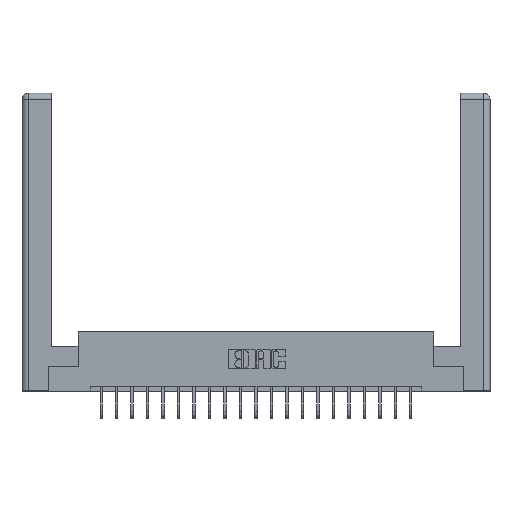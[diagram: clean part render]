
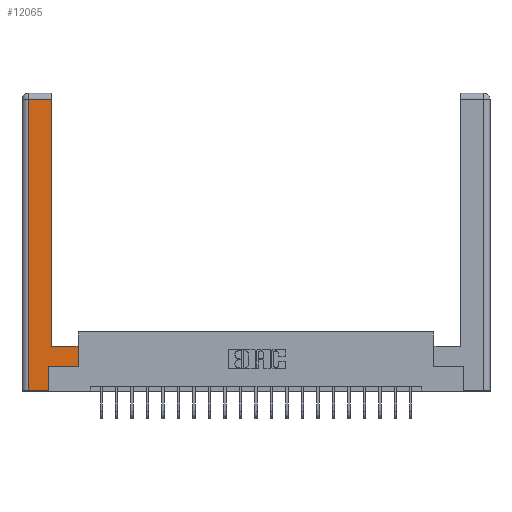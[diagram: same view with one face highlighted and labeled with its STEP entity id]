
A CAD part, top view. The second image highlights one B-rep face of the part: STEP entity #12065.
In plain terms, the highlighted planar face has unit normal (0, 0, 1).
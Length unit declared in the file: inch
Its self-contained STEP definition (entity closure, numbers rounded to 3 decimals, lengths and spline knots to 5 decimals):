
#113 = DIRECTION ( 'NONE',  ( 1., 0., 0. ) ) ;
#140 = CARTESIAN_POINT ( 'NONE',  ( 0.565, 0.45, 0. ) ) ;
#255 = PLANE ( 'NONE',  #15742 ) ;
#606 = CARTESIAN_POINT ( 'NONE',  ( 0.565, 0.245, 0. ) ) ;
#1697 = VERTEX_POINT ( 'NONE', #17633 ) ;
#1899 = VECTOR ( 'NONE', #22038, 39.37008 ) ;
#2042 = CARTESIAN_POINT ( 'NONE',  ( 0.265, 0.245, 0. ) ) ;
#2050 = CARTESIAN_POINT ( 'NONE',  ( 0.565, 0.245, 0. ) ) ;
#2191 = ORIENTED_EDGE ( 'NONE', *, *, #4860, .T. ) ;
#2798 = VECTOR ( 'NONE', #8363, 39.37008 ) ;
#2840 = LINE ( 'NONE', #2050, #11874 ) ;
#4106 = DIRECTION ( 'NONE',  ( 0., 0., -1. ) ) ;
#4717 = CARTESIAN_POINT ( 'NONE',  ( 0.0615, 0., 0. ) ) ;
#4752 = DIRECTION ( 'NONE',  ( 1., 0., 0. ) ) ;
#4832 = CARTESIAN_POINT ( 'NONE',  ( 0.265, 0.245, 0. ) ) ;
#4838 = VERTEX_POINT ( 'NONE', #606 ) ;
#4860 = EDGE_CURVE ( 'NONE', #20187, #1697, #8771, .T. ) ;
#6125 = DIRECTION ( 'NONE',  ( 0., 1., 0. ) ) ;
#6168 = EDGE_CURVE ( 'NONE', #13721, #4838, #2840, .T. ) ;
#6386 = VECTOR ( 'NONE', #6125, 39.37008 ) ;
#6642 = LINE ( 'NONE', #4717, #18558 ) ;
#7046 = ORIENTED_EDGE ( 'NONE', *, *, #20516, .T. ) ;
#7516 = LINE ( 'NONE', #4832, #6386 ) ;
#7944 = DIRECTION ( 'NONE',  ( 0., 1., 0. ) ) ;
#8049 = ORIENTED_EDGE ( 'NONE', *, *, #19619, .T. ) ;
#8363 = DIRECTION ( 'NONE',  ( -1., 0., 0. ) ) ;
#8366 = VERTEX_POINT ( 'NONE', #10975 ) ;
#8700 = EDGE_LOOP ( 'NONE', ( #2191, #8049, #17973, #20646, #8934, #20137, #7046, #23419 ) ) ;
#8736 = VERTEX_POINT ( 'NONE', #13811 ) ;
#8771 = LINE ( 'NONE', #22196, #15490 ) ;
#8934 = ORIENTED_EDGE ( 'NONE', *, *, #19689, .T. ) ;
#10246 = CARTESIAN_POINT ( 'NONE',  ( 0.295, 0.45, 0. ) ) ;
#10975 = CARTESIAN_POINT ( 'NONE',  ( 0.0615, 0., 0. ) ) ;
#11301 = LINE ( 'NONE', #21225, #18965 ) ;
#11869 = EDGE_CURVE ( 'NONE', #8366, #14856, #11301, .T. ) ;
#11874 = VECTOR ( 'NONE', #113, 39.37008 ) ;
#11919 = DIRECTION ( 'NONE',  ( 0., -1., 0. ) ) ;
#12065 = ADVANCED_FACE ( 'NONE', ( #15791 ), #255, .F. ) ;
#12980 = CARTESIAN_POINT ( 'NONE',  ( 0.565, 0.45, 0. ) ) ;
#13107 = VECTOR ( 'NONE', #14637, 39.37008 ) ;
#13721 = VERTEX_POINT ( 'NONE', #2042 ) ;
#13811 = CARTESIAN_POINT ( 'NONE',  ( 0.0615, 2.94, 0. ) ) ;
#14637 = DIRECTION ( 'NONE',  ( 0., 1., 0. ) ) ;
#14856 = VERTEX_POINT ( 'NONE', #22261 ) ;
#15490 = VECTOR ( 'NONE', #7944, 39.37008 ) ;
#15742 = AXIS2_PLACEMENT_3D ( 'NONE', #21913, #4106, #21996 ) ;
#15791 = FACE_OUTER_BOUND ( 'NONE', #8700, .T. ) ;
#17633 = CARTESIAN_POINT ( 'NONE',  ( 0.295, 2.94, 0. ) ) ;
#17711 = LINE ( 'NONE', #18644, #1899 ) ;
#17783 = LINE ( 'NONE', #10246, #2798 ) ;
#17973 = ORIENTED_EDGE ( 'NONE', *, *, #20295, .T. ) ;
#18558 = VECTOR ( 'NONE', #11919, 39.37008 ) ;
#18644 = CARTESIAN_POINT ( 'NONE',  ( 0.0615, 2.94, 0. ) ) ;
#18805 = VERTEX_POINT ( 'NONE', #12980 ) ;
#18965 = VECTOR ( 'NONE', #4752, 39.37008 ) ;
#19619 = EDGE_CURVE ( 'NONE', #1697, #8736, #17711, .T. ) ;
#19689 = EDGE_CURVE ( 'NONE', #14856, #13721, #7516, .T. ) ;
#20137 = ORIENTED_EDGE ( 'NONE', *, *, #6168, .T. ) ;
#20187 = VERTEX_POINT ( 'NONE', #21095 ) ;
#20295 = EDGE_CURVE ( 'NONE', #8736, #8366, #6642, .T. ) ;
#20516 = EDGE_CURVE ( 'NONE', #4838, #18805, #23074, .T. ) ;
#20646 = ORIENTED_EDGE ( 'NONE', *, *, #11869, .T. ) ;
#21095 = CARTESIAN_POINT ( 'NONE',  ( 0.295, 0.45, 0. ) ) ;
#21225 = CARTESIAN_POINT ( 'NONE',  ( 0.265, 0., 0. ) ) ;
#21610 = EDGE_CURVE ( 'NONE', #18805, #20187, #17783, .T. ) ;
#21913 = CARTESIAN_POINT ( 'NONE',  ( 0., 0., 0. ) ) ;
#21996 = DIRECTION ( 'NONE',  ( -1., 0., 0. ) ) ;
#22038 = DIRECTION ( 'NONE',  ( -1., 0., 0. ) ) ;
#22196 = CARTESIAN_POINT ( 'NONE',  ( 0.295, 3., 0. ) ) ;
#22261 = CARTESIAN_POINT ( 'NONE',  ( 0.265, 0., 0. ) ) ;
#23074 = LINE ( 'NONE', #140, #13107 ) ;
#23419 = ORIENTED_EDGE ( 'NONE', *, *, #21610, .T. ) ;
